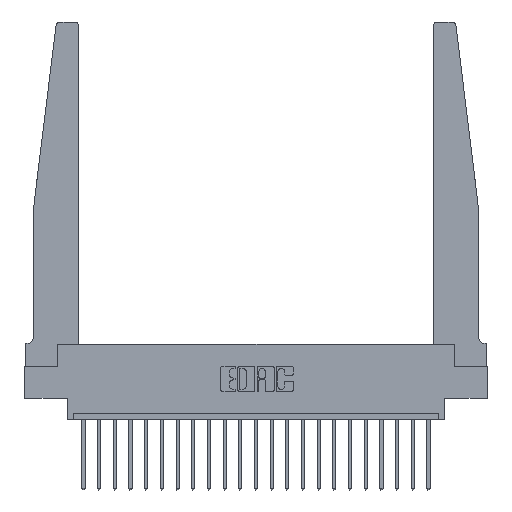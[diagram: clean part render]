
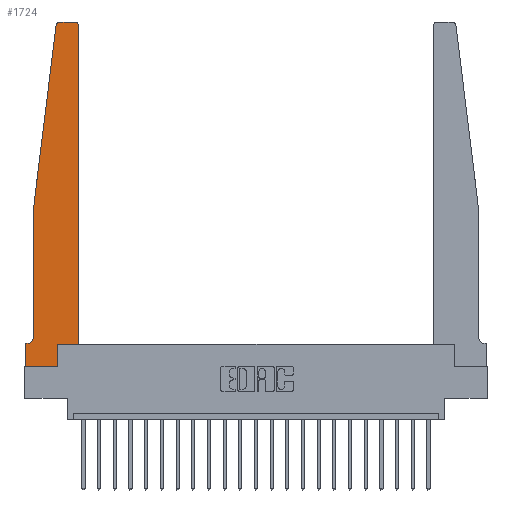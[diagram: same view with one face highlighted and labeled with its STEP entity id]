
A CAD part, top view. The second image highlights one B-rep face of the part: STEP entity #1724.
In plain terms, the highlighted planar face has unit normal (0, 0, 1).
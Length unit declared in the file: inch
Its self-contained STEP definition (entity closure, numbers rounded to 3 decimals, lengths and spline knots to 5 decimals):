
#68 = PLANE ( 'NONE',  #224 ) ;
#90 = VECTOR ( 'NONE', #21082, 39.37008 ) ;
#202 = VECTOR ( 'NONE', #11189, 39.37008 ) ;
#224 = AXIS2_PLACEMENT_3D ( 'NONE', #19016, #3667, #1977 ) ;
#689 = EDGE_CURVE ( 'NONE', #18458, #10415, #6100, .T. ) ;
#1008 = CARTESIAN_POINT ( 'NONE',  ( 0.425, 0.18, 0.37 ) ) ;
#1245 = VERTEX_POINT ( 'NONE', #12228 ) ;
#1724 = ADVANCED_FACE ( 'NONE', ( #5358 ), #68, .T. ) ;
#1977 = DIRECTION ( 'NONE',  ( 1., 0., 0. ) ) ;
#2845 = EDGE_CURVE ( 'NONE', #5702, #17782, #3226, .T. ) ;
#2910 = CARTESIAN_POINT ( 'NONE',  ( 0.425, 0.18, 0.37 ) ) ;
#3013 = LINE ( 'NONE', #18593, #18516 ) ;
#3226 = LINE ( 'NONE', #10092, #13171 ) ;
#3244 = CARTESIAN_POINT ( 'NONE',  ( 0.395, 2.72, 0.37 ) ) ;
#3362 = DIRECTION ( 'NONE',  ( 1., 0., 0. ) ) ;
#3667 = DIRECTION ( 'NONE',  ( 0., 0., 1. ) ) ;
#4021 = VERTEX_POINT ( 'NONE', #19177 ) ;
#4398 = EDGE_CURVE ( 'NONE', #16189, #7565, #5806, .T. ) ;
#4448 = DIRECTION ( 'NONE',  ( 0., 0., -1. ) ) ;
#4528 = AXIS2_PLACEMENT_3D ( 'NONE', #18240, #4448, #21359 ) ;
#4790 = DIRECTION ( 'NONE',  ( 1., 0., 0. ) ) ;
#4816 = DIRECTION ( 'NONE',  ( 1., 0., 0. ) ) ;
#5060 = EDGE_LOOP ( 'NONE', ( #19691, #14359, #8718, #6079, #10705, #8907, #7404, #10322, #17723, #8506, #15560, #7295 ) ) ;
#5358 = FACE_OUTER_BOUND ( 'NONE', #5060, .T. ) ;
#5592 = DIRECTION ( 'NONE',  ( 0., -1., 0. ) ) ;
#5702 = VERTEX_POINT ( 'NONE', #18949 ) ;
#5806 = LINE ( 'NONE', #20946, #14066 ) ;
#5958 = CIRCLE ( 'NONE', #4528, 0.05 ) ;
#6079 = ORIENTED_EDGE ( 'NONE', *, *, #689, .T. ) ;
#6100 = LINE ( 'NONE', #16545, #11914 ) ;
#7041 = CARTESIAN_POINT ( 'NONE',  ( 0.2605, 0.18, 0.37 ) ) ;
#7295 = ORIENTED_EDGE ( 'NONE', *, *, #16044, .T. ) ;
#7404 = ORIENTED_EDGE ( 'NONE', *, *, #4398, .T. ) ;
#7441 = EDGE_CURVE ( 'NONE', #10415, #18023, #5958, .T. ) ;
#7565 = VERTEX_POINT ( 'NONE', #17406 ) ;
#7568 = LINE ( 'NONE', #19778, #18824 ) ;
#7575 = CARTESIAN_POINT ( 'NONE',  ( 0., 0., 0.37 ) ) ;
#7595 = CARTESIAN_POINT ( 'NONE',  ( 0., 0.1875, 0.37 ) ) ;
#7806 = CARTESIAN_POINT ( 'NONE',  ( 0.27653, 2.75, 0.37 ) ) ;
#8399 = CARTESIAN_POINT ( 'NONE',  ( 0.27653, 2.72, 0.37 ) ) ;
#8506 = ORIENTED_EDGE ( 'NONE', *, *, #17681, .T. ) ;
#8718 = ORIENTED_EDGE ( 'NONE', *, *, #13242, .T. ) ;
#8907 = ORIENTED_EDGE ( 'NONE', *, *, #14429, .T. ) ;
#9185 = CARTESIAN_POINT ( 'NONE',  ( 0.065, 1.25, 0.37 ) ) ;
#9837 = DIRECTION ( 'NONE',  ( 0., -1., 0. ) ) ;
#10092 = CARTESIAN_POINT ( 'NONE',  ( 0.2605, 0.18, 0.37 ) ) ;
#10155 = VERTEX_POINT ( 'NONE', #12301 ) ;
#10189 = EDGE_CURVE ( 'NONE', #7565, #5702, #15757, .T. ) ;
#10322 = ORIENTED_EDGE ( 'NONE', *, *, #10189, .T. ) ;
#10415 = VERTEX_POINT ( 'NONE', #16962 ) ;
#10694 = EDGE_CURVE ( 'NONE', #20125, #10155, #19721, .T. ) ;
#10705 = ORIENTED_EDGE ( 'NONE', *, *, #7441, .T. ) ;
#11064 = DIRECTION ( 'NONE',  ( -0.122, -0.992, 0. ) ) ;
#11189 = DIRECTION ( 'NONE',  ( -1., 0., 0. ) ) ;
#11528 = DIRECTION ( 'NONE',  ( 0., 0., 1. ) ) ;
#11748 = VERTEX_POINT ( 'NONE', #7806 ) ;
#11914 = VECTOR ( 'NONE', #9837, 39.37008 ) ;
#12093 = CARTESIAN_POINT ( 'NONE',  ( 0.015, 0.1875, 0.37 ) ) ;
#12228 = CARTESIAN_POINT ( 'NONE',  ( 0.24675, 2.72367, 0.37 ) ) ;
#12301 = CARTESIAN_POINT ( 'NONE',  ( 0.425, 2.72, 0.37 ) ) ;
#12370 = CARTESIAN_POINT ( 'NONE',  ( 0.065, 1.25, 0.37 ) ) ;
#12610 = DIRECTION ( 'NONE',  ( 1., 0., 0. ) ) ;
#12701 = VECTOR ( 'NONE', #11064, 39.37008 ) ;
#12788 = CIRCLE ( 'NONE', #13146, 0.03 ) ;
#13146 = AXIS2_PLACEMENT_3D ( 'NONE', #3244, #18712, #3362 ) ;
#13171 = VECTOR ( 'NONE', #16907, 39.37008 ) ;
#13242 = EDGE_CURVE ( 'NONE', #1245, #18458, #17673, .T. ) ;
#14066 = VECTOR ( 'NONE', #5592, 39.37008 ) ;
#14359 = ORIENTED_EDGE ( 'NONE', *, *, #19110, .T. ) ;
#14429 = EDGE_CURVE ( 'NONE', #18023, #16189, #21363, .T. ) ;
#14553 = CARTESIAN_POINT ( 'NONE',  ( 0.065, 0.1875, 0.37 ) ) ;
#14791 = EDGE_CURVE ( 'NONE', #4021, #11748, #7568, .T. ) ;
#15560 = ORIENTED_EDGE ( 'NONE', *, *, #10694, .T. ) ;
#15757 = LINE ( 'NONE', #7575, #16966 ) ;
#16035 = AXIS2_PLACEMENT_3D ( 'NONE', #8399, #11528, #4790 ) ;
#16044 = EDGE_CURVE ( 'NONE', #10155, #4021, #12788, .T. ) ;
#16189 = VERTEX_POINT ( 'NONE', #7595 ) ;
#16545 = CARTESIAN_POINT ( 'NONE',  ( 0.065, 1.25, 0.37 ) ) ;
#16907 = DIRECTION ( 'NONE',  ( 0., 1., 0. ) ) ;
#16962 = CARTESIAN_POINT ( 'NONE',  ( 0.065, 0.2375, 0.37 ) ) ;
#16966 = VECTOR ( 'NONE', #12610, 39.37008 ) ;
#17406 = CARTESIAN_POINT ( 'NONE',  ( 0., 0., 0.37 ) ) ;
#17655 = DIRECTION ( 'NONE',  ( -1., 0., 0. ) ) ;
#17673 = LINE ( 'NONE', #9185, #12701 ) ;
#17681 = EDGE_CURVE ( 'NONE', #17782, #20125, #3013, .T. ) ;
#17723 = ORIENTED_EDGE ( 'NONE', *, *, #2845, .T. ) ;
#17782 = VERTEX_POINT ( 'NONE', #7041 ) ;
#18023 = VERTEX_POINT ( 'NONE', #12093 ) ;
#18177 = CIRCLE ( 'NONE', #16035, 0.03 ) ;
#18240 = CARTESIAN_POINT ( 'NONE',  ( 0.015, 0.2375, 0.37 ) ) ;
#18458 = VERTEX_POINT ( 'NONE', #12370 ) ;
#18516 = VECTOR ( 'NONE', #4816, 39.37008 ) ;
#18593 = CARTESIAN_POINT ( 'NONE',  ( 0.425, 0.18, 0.37 ) ) ;
#18712 = DIRECTION ( 'NONE',  ( 0., 0., 1. ) ) ;
#18824 = VECTOR ( 'NONE', #17655, 39.37008 ) ;
#18949 = CARTESIAN_POINT ( 'NONE',  ( 0.2605, 0., 0.37 ) ) ;
#19016 = CARTESIAN_POINT ( 'NONE',  ( 0., 0.1875, 0.37 ) ) ;
#19110 = EDGE_CURVE ( 'NONE', #11748, #1245, #18177, .T. ) ;
#19177 = CARTESIAN_POINT ( 'NONE',  ( 0.395, 2.75, 0.37 ) ) ;
#19691 = ORIENTED_EDGE ( 'NONE', *, *, #14791, .T. ) ;
#19721 = LINE ( 'NONE', #1008, #90 ) ;
#19778 = CARTESIAN_POINT ( 'NONE',  ( 0.25, 2.75, 0.37 ) ) ;
#20125 = VERTEX_POINT ( 'NONE', #2910 ) ;
#20946 = CARTESIAN_POINT ( 'NONE',  ( 0., 0., 0.37 ) ) ;
#21082 = DIRECTION ( 'NONE',  ( 0., 1., 0. ) ) ;
#21359 = DIRECTION ( 'NONE',  ( -1., 0., 0. ) ) ;
#21363 = LINE ( 'NONE', #14553, #202 ) ;
